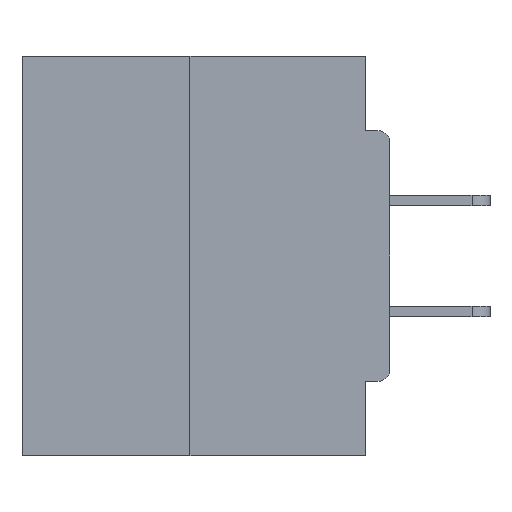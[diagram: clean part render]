
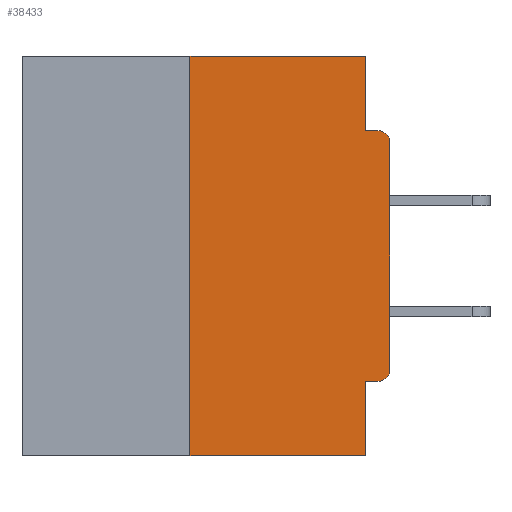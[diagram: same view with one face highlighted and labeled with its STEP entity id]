
A CAD part, left-side view. The second image highlights one B-rep face of the part: STEP entity #38433.
In plain terms, the highlighted planar face has unit normal (-1, 0, 0).
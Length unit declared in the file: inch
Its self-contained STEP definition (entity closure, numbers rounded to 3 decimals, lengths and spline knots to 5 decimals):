
#182 = VECTOR ( 'NONE', #29688, 39.37008 ) ;
#435 = EDGE_CURVE ( 'NONE', #33922, #31737, #18771, .T. ) ;
#464 = DIRECTION ( 'NONE',  ( -1., 0., 0. ) ) ;
#581 = DIRECTION ( 'NONE',  ( 0., 0., 1. ) ) ;
#1339 = ORIENTED_EDGE ( 'NONE', *, *, #12935, .F. ) ;
#2168 = ORIENTED_EDGE ( 'NONE', *, *, #13464, .F. ) ;
#2615 = VECTOR ( 'NONE', #18513, 39.37008 ) ;
#2910 = CARTESIAN_POINT ( 'NONE',  ( 0., 0.015, -0.1085 ) ) ;
#3578 = EDGE_CURVE ( 'NONE', #8742, #20474, #8642, .T. ) ;
#3980 = DIRECTION ( 'NONE',  ( 0., 0., -1. ) ) ;
#3999 = CARTESIAN_POINT ( 'NONE',  ( 0., 0.015, -0.4065 ) ) ;
#4243 = VECTOR ( 'NONE', #581, 39.37008 ) ;
#5244 = LINE ( 'NONE', #35323, #4243 ) ;
#5615 = CARTESIAN_POINT ( 'NONE',  ( 0., 0., -0.1085 ) ) ;
#5751 = CARTESIAN_POINT ( 'NONE',  ( 0., 0.46, 0. ) ) ;
#5991 = DIRECTION ( 'NONE',  ( -1., 0., 0. ) ) ;
#6123 = DIRECTION ( 'NONE',  ( 0., 0., -1. ) ) ;
#7051 = ORIENTED_EDGE ( 'NONE', *, *, #29974, .T. ) ;
#7207 = CARTESIAN_POINT ( 'NONE',  ( 0., 0.015, -0.3915 ) ) ;
#7621 = CARTESIAN_POINT ( 'NONE',  ( 0., 0.031, 0. ) ) ;
#8348 = CARTESIAN_POINT ( 'NONE',  ( 0., 0.25, 0. ) ) ;
#8368 = AXIS2_PLACEMENT_3D ( 'NONE', #2910, #5991, #6123 ) ;
#8499 = CARTESIAN_POINT ( 'NONE',  ( 0., 0.031, -0.5 ) ) ;
#8606 = VECTOR ( 'NONE', #36122, 39.37008 ) ;
#8642 = CIRCLE ( 'NONE', #23904, 0.015 ) ;
#8686 = VERTEX_POINT ( 'NONE', #7621 ) ;
#8742 = VERTEX_POINT ( 'NONE', #3999 ) ;
#10402 = VERTEX_POINT ( 'NONE', #8348 ) ;
#10678 = EDGE_CURVE ( 'NONE', #33922, #10402, #5244, .T. ) ;
#12152 = CARTESIAN_POINT ( 'NONE',  ( 0., 0.015, -0.0935 ) ) ;
#12507 = VERTEX_POINT ( 'NONE', #5615 ) ;
#12566 = EDGE_CURVE ( 'NONE', #10402, #8686, #24670, .T. ) ;
#12935 = EDGE_CURVE ( 'NONE', #39697, #30297, #23626, .T. ) ;
#13464 = EDGE_CURVE ( 'NONE', #8686, #39697, #38090, .T. ) ;
#13498 = DIRECTION ( 'NONE',  ( 1., 0., 0. ) ) ;
#14124 = CARTESIAN_POINT ( 'NONE',  ( 0., 0.031, 0. ) ) ;
#15278 = LINE ( 'NONE', #31366, #23769 ) ;
#15568 = VECTOR ( 'NONE', #36509, 39.37008 ) ;
#16217 = VECTOR ( 'NONE', #29761, 39.37008 ) ;
#16516 = VECTOR ( 'NONE', #37453, 39.37008 ) ;
#18513 = DIRECTION ( 'NONE',  ( 0., -1., 0. ) ) ;
#18768 = EDGE_LOOP ( 'NONE', ( #28051, #31322, #27542, #33713, #25131, #22943, #7051, #22623, #1339, #2168 ) ) ;
#18771 = LINE ( 'NONE', #22759, #182 ) ;
#20169 = CARTESIAN_POINT ( 'NONE',  ( 0., 0., 0. ) ) ;
#20474 = VERTEX_POINT ( 'NONE', #21614 ) ;
#20692 = CIRCLE ( 'NONE', #8368, 0.015 ) ;
#21614 = CARTESIAN_POINT ( 'NONE',  ( 0., 0., -0.3915 ) ) ;
#22251 = LINE ( 'NONE', #20169, #16217 ) ;
#22623 = ORIENTED_EDGE ( 'NONE', *, *, #31378, .T. ) ;
#22759 = CARTESIAN_POINT ( 'NONE',  ( 0., 0.46, -0.5 ) ) ;
#22943 = ORIENTED_EDGE ( 'NONE', *, *, #3578, .T. ) ;
#22993 = CARTESIAN_POINT ( 'NONE',  ( 0., 0.031, -0.0935 ) ) ;
#23026 = AXIS2_PLACEMENT_3D ( 'NONE', #32631, #13498, #35864 ) ;
#23030 = PLANE ( 'NONE',  #23026 ) ;
#23150 = CARTESIAN_POINT ( 'NONE',  ( 0., 0., -0.0935 ) ) ;
#23626 = LINE ( 'NONE', #23150, #8606 ) ;
#23769 = VECTOR ( 'NONE', #24104, 39.37008 ) ;
#23904 = AXIS2_PLACEMENT_3D ( 'NONE', #7207, #464, #3980 ) ;
#24104 = DIRECTION ( 'NONE',  ( 0., 0., -1. ) ) ;
#24670 = LINE ( 'NONE', #5751, #2615 ) ;
#24854 = EDGE_CURVE ( 'NONE', #8742, #34744, #41079, .T. ) ;
#25131 = ORIENTED_EDGE ( 'NONE', *, *, #24854, .F. ) ;
#27542 = ORIENTED_EDGE ( 'NONE', *, *, #435, .T. ) ;
#27544 = CARTESIAN_POINT ( 'NONE',  ( 0., 0.031, -0.4065 ) ) ;
#28051 = ORIENTED_EDGE ( 'NONE', *, *, #12566, .F. ) ;
#28302 = EDGE_CURVE ( 'NONE', #34744, #31737, #15278, .T. ) ;
#29688 = DIRECTION ( 'NONE',  ( 0., -1., 0. ) ) ;
#29761 = DIRECTION ( 'NONE',  ( 0., 0., 1. ) ) ;
#29807 = FACE_OUTER_BOUND ( 'NONE', #18768, .T. ) ;
#29974 = EDGE_CURVE ( 'NONE', #20474, #12507, #22251, .T. ) ;
#30297 = VERTEX_POINT ( 'NONE', #12152 ) ;
#30817 = CARTESIAN_POINT ( 'NONE',  ( 0., 0., -0.4065 ) ) ;
#31322 = ORIENTED_EDGE ( 'NONE', *, *, #10678, .F. ) ;
#31366 = CARTESIAN_POINT ( 'NONE',  ( 0., 0.031, -0.5 ) ) ;
#31378 = EDGE_CURVE ( 'NONE', #12507, #30297, #20692, .T. ) ;
#31737 = VERTEX_POINT ( 'NONE', #8499 ) ;
#32631 = CARTESIAN_POINT ( 'NONE',  ( 0., 0.46, 0. ) ) ;
#33622 = CARTESIAN_POINT ( 'NONE',  ( 0., 0.25, -0.5 ) ) ;
#33713 = ORIENTED_EDGE ( 'NONE', *, *, #28302, .F. ) ;
#33922 = VERTEX_POINT ( 'NONE', #33622 ) ;
#34744 = VERTEX_POINT ( 'NONE', #27544 ) ;
#35323 = CARTESIAN_POINT ( 'NONE',  ( 0., 0.25, 0. ) ) ;
#35864 = DIRECTION ( 'NONE',  ( 0., 0., -1. ) ) ;
#36122 = DIRECTION ( 'NONE',  ( 0., -1., 0. ) ) ;
#36509 = DIRECTION ( 'NONE',  ( 0., 0., -1. ) ) ;
#37453 = DIRECTION ( 'NONE',  ( 0., 1., 0. ) ) ;
#38090 = LINE ( 'NONE', #14124, #15568 ) ;
#38433 = ADVANCED_FACE ( 'NONE', ( #29807 ), #23030, .F. ) ;
#39697 = VERTEX_POINT ( 'NONE', #22993 ) ;
#41079 = LINE ( 'NONE', #30817, #16516 ) ;
